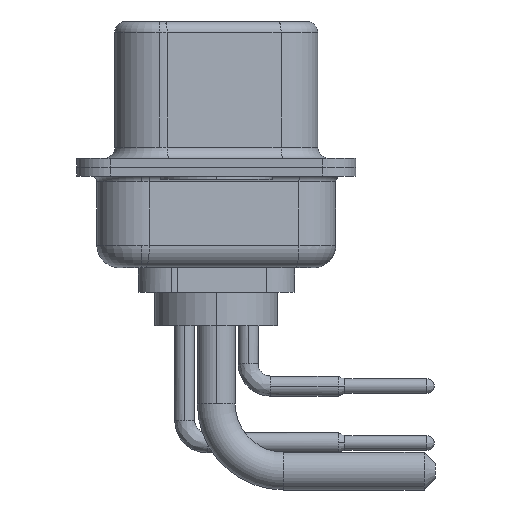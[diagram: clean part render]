
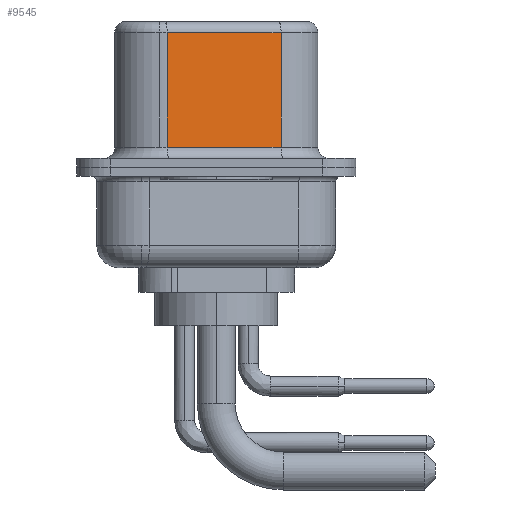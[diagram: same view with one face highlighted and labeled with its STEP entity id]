
A CAD part, left-side view. The second image highlights one B-rep face of the part: STEP entity #9545.
In plain terms, the highlighted planar face has unit normal (-0.985, -0.174, 0).
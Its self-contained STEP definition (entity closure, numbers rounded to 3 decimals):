
#172 = DIRECTION ( 'NONE',  ( -0.174, 0.985, 0. ) ) ;
#897 = DIRECTION ( 'NONE',  ( -0.174, 0.985, 0. ) ) ;
#2276 = LINE ( 'NONE', #12726, #5669 ) ;
#2984 = CARTESIAN_POINT ( 'NONE',  ( 4.58, -2.897, 6.52 ) ) ;
#3546 = CARTESIAN_POINT ( 'NONE',  ( 3.68, 2.203, 0.9 ) ) ;
#3732 = EDGE_CURVE ( 'NONE', #18707, #5595, #13399, .T. ) ;
#3796 = CARTESIAN_POINT ( 'NONE',  ( 4.58, -2.897, 6.02 ) ) ;
#3909 = CARTESIAN_POINT ( 'NONE',  ( 3.68, 2.203, 6.02 ) ) ;
#4271 = EDGE_LOOP ( 'NONE', ( #20683, #19322, #18994, #8335 ) ) ;
#5595 = VERTEX_POINT ( 'NONE', #3546 ) ;
#5669 = VECTOR ( 'NONE', #17709, 1000. ) ;
#6047 = EDGE_CURVE ( 'NONE', #9154, #9779, #19953, .T. ) ;
#6355 = VECTOR ( 'NONE', #20017, 1000. ) ;
#6578 = CARTESIAN_POINT ( 'NONE',  ( 3.68, 2.203, 6.52 ) ) ;
#8187 = EDGE_CURVE ( 'NONE', #9154, #18707, #15139, .T. ) ;
#8335 = ORIENTED_EDGE ( 'NONE', *, *, #14572, .T. ) ;
#9154 = VERTEX_POINT ( 'NONE', #12440 ) ;
#9381 = FACE_OUTER_BOUND ( 'NONE', #4271, .T. ) ;
#9545 = ADVANCED_FACE ( 'NONE', ( #9381 ), #17770, .F. ) ;
#9705 = DIRECTION ( 'NONE',  ( 0., 0., -1. ) ) ;
#9779 = VERTEX_POINT ( 'NONE', #10347 ) ;
#10347 = CARTESIAN_POINT ( 'NONE',  ( 4.58, -2.897, 0.9 ) ) ;
#12440 = CARTESIAN_POINT ( 'NONE',  ( 4.58, -2.897, 6.02 ) ) ;
#12726 = CARTESIAN_POINT ( 'NONE',  ( 4.58, -2.897, 0.9 ) ) ;
#13399 = LINE ( 'NONE', #6578, #6355 ) ;
#14572 = EDGE_CURVE ( 'NONE', #5595, #9779, #2276, .T. ) ;
#14900 = AXIS2_PLACEMENT_3D ( 'NONE', #16090, #21288, #897 ) ;
#15139 = LINE ( 'NONE', #3796, #18785 ) ;
#16090 = CARTESIAN_POINT ( 'NONE',  ( 4.58, -2.897, 6.52 ) ) ;
#17709 = DIRECTION ( 'NONE',  ( 0.174, -0.985, 0. ) ) ;
#17770 = PLANE ( 'NONE',  #14900 ) ;
#18707 = VERTEX_POINT ( 'NONE', #3909 ) ;
#18785 = VECTOR ( 'NONE', #172, 1000. ) ;
#18994 = ORIENTED_EDGE ( 'NONE', *, *, #3732, .T. ) ;
#19322 = ORIENTED_EDGE ( 'NONE', *, *, #8187, .T. ) ;
#19953 = LINE ( 'NONE', #2984, #20810 ) ;
#20017 = DIRECTION ( 'NONE',  ( 0., 0., -1. ) ) ;
#20683 = ORIENTED_EDGE ( 'NONE', *, *, #6047, .F. ) ;
#20810 = VECTOR ( 'NONE', #9705, 1000. ) ;
#21288 = DIRECTION ( 'NONE',  ( 0.985, 0.174, 0. ) ) ;
